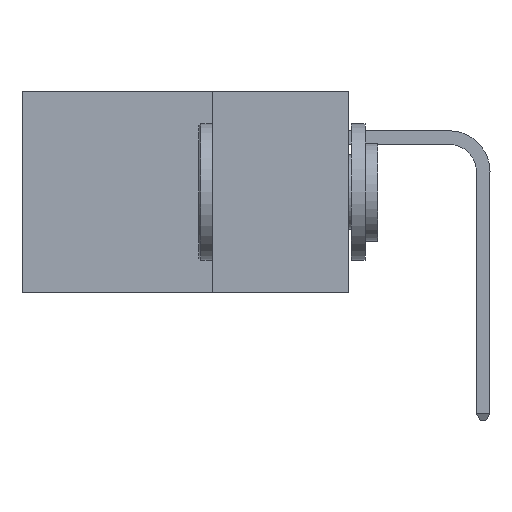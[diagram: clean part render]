
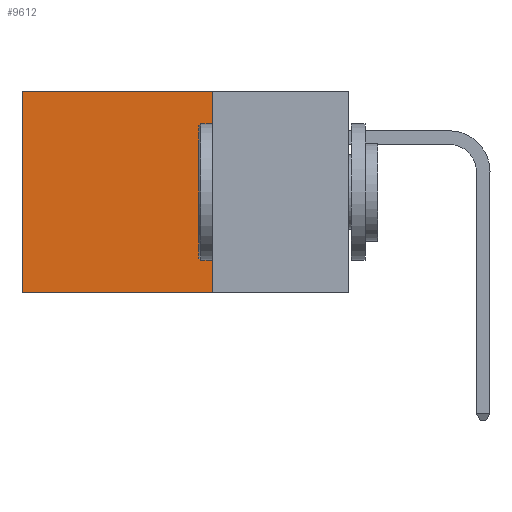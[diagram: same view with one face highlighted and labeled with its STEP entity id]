
A CAD part, left-side view. The second image highlights one B-rep face of the part: STEP entity #9612.
In plain terms, the highlighted planar face has unit normal (-1, 0, 0).
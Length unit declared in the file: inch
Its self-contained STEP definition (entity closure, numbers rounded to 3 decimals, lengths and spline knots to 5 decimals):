
#67 = DIRECTION ( 'NONE',  ( 0., 0., -1. ) ) ;
#173 = EDGE_CURVE ( 'NONE', #8049, #11753, #1806, .T. ) ;
#306 = CARTESIAN_POINT ( 'NONE',  ( 0.2875, 0.25, 0. ) ) ;
#378 = DIRECTION ( 'NONE',  ( 1., 0., 0. ) ) ;
#1456 = CARTESIAN_POINT ( 'NONE',  ( 0.2875, 0.25, 0. ) ) ;
#1806 = LINE ( 'NONE', #7953, #6717 ) ;
#3562 = VECTOR ( 'NONE', #12589, 39.37008 ) ;
#3658 = CARTESIAN_POINT ( 'NONE',  ( 0.2875, 0.25, -0.37 ) ) ;
#4090 = ORIENTED_EDGE ( 'NONE', *, *, #173, .T. ) ;
#4481 = CARTESIAN_POINT ( 'NONE',  ( 0.2875, 0.25, 0. ) ) ;
#4537 = CARTESIAN_POINT ( 'NONE',  ( 0.2875, 0.25, -0.37 ) ) ;
#5038 = EDGE_CURVE ( 'NONE', #15714, #9907, #7018, .T. ) ;
#5878 = CARTESIAN_POINT ( 'NONE',  ( 0.2875, 0.6, 0. ) ) ;
#6260 = EDGE_LOOP ( 'NONE', ( #4090, #20261, #14297, #9372 ) ) ;
#6717 = VECTOR ( 'NONE', #67, 39.37008 ) ;
#7018 = LINE ( 'NONE', #4481, #14326 ) ;
#7384 = LINE ( 'NONE', #1456, #3562 ) ;
#7392 = EDGE_CURVE ( 'NONE', #9907, #11753, #13267, .T. ) ;
#7953 = CARTESIAN_POINT ( 'NONE',  ( 0.2875, 0.6, 0. ) ) ;
#8049 = VERTEX_POINT ( 'NONE', #5878 ) ;
#9372 = ORIENTED_EDGE ( 'NONE', *, *, #10001, .T. ) ;
#9571 = AXIS2_PLACEMENT_3D ( 'NONE', #306, #378, #11580 ) ;
#9612 = ADVANCED_FACE ( 'NONE', ( #19360 ), #17893, .F. ) ;
#9635 = VECTOR ( 'NONE', #13074, 39.37008 ) ;
#9907 = VERTEX_POINT ( 'NONE', #4537 ) ;
#10001 = EDGE_CURVE ( 'NONE', #15714, #8049, #7384, .T. ) ;
#11580 = DIRECTION ( 'NONE',  ( 0., 0., -1. ) ) ;
#11753 = VERTEX_POINT ( 'NONE', #20542 ) ;
#12589 = DIRECTION ( 'NONE',  ( 0., 1., 0. ) ) ;
#13074 = DIRECTION ( 'NONE',  ( 0., 1., 0. ) ) ;
#13267 = LINE ( 'NONE', #3658, #9635 ) ;
#14297 = ORIENTED_EDGE ( 'NONE', *, *, #5038, .F. ) ;
#14326 = VECTOR ( 'NONE', #17081, 39.37008 ) ;
#15714 = VERTEX_POINT ( 'NONE', #20215 ) ;
#17081 = DIRECTION ( 'NONE',  ( 0., 0., -1. ) ) ;
#17893 = PLANE ( 'NONE',  #9571 ) ;
#19360 = FACE_OUTER_BOUND ( 'NONE', #6260, .T. ) ;
#20215 = CARTESIAN_POINT ( 'NONE',  ( 0.2875, 0.25, 0. ) ) ;
#20261 = ORIENTED_EDGE ( 'NONE', *, *, #7392, .F. ) ;
#20542 = CARTESIAN_POINT ( 'NONE',  ( 0.2875, 0.6, -0.37 ) ) ;
